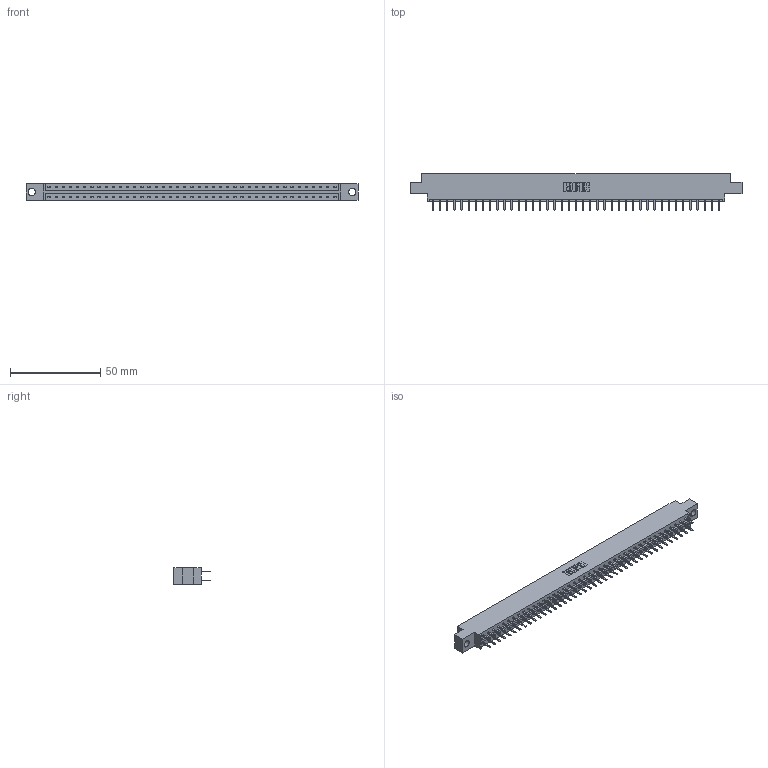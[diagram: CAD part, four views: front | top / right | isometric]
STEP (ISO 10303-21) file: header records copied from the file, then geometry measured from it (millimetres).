
FILE_DESCRIPTION (( 'STEP AP203' ), '1' );
FILE_NAME ('833-082-520-804.STEP', '2020-06-05T23:04:48', ( '' ), ( '' ), 'SwSTEP 2.0', 'SolidWorks 2020', '' );
FILE_SCHEMA (( 'CONFIG_CONTROL_DESIGN' ));
Length unit declared in the file: inch
Products named in the file (3): 345-292-001_345-293-120; 833 Part_Offset - .156 Dia - TH; 833-082-520-804
Assembly tree (83 placements, depth 2):
  833-082-520-804
    833 Part_Offset - .156 Dia - TH
    345-292-001_345-293-120  x82
Bounding box: 184 x 20.02 x 9.4 mm (x, y, z)
Volume: 18424.1 mm3; surface area: 21695.8 mm2
Topology: 83 solids, 83 shells, 4710 faces, 13689 edges, 8906 vertices
Faces by surface type: plane 3190, cylinder 1520
Entity records: 26755 total; most frequent: CARTESIAN_POINT 4450, ORIENTED_EDGE 4374, DIRECTION 3791, EDGE_CURVE 2187, LINE 2055, VECTOR 2055, VERTEX_POINT 1454, AXIS2_PLACEMENT_3D 868
